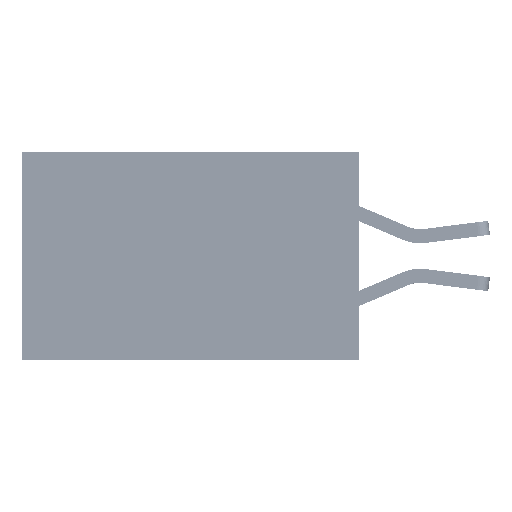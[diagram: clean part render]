
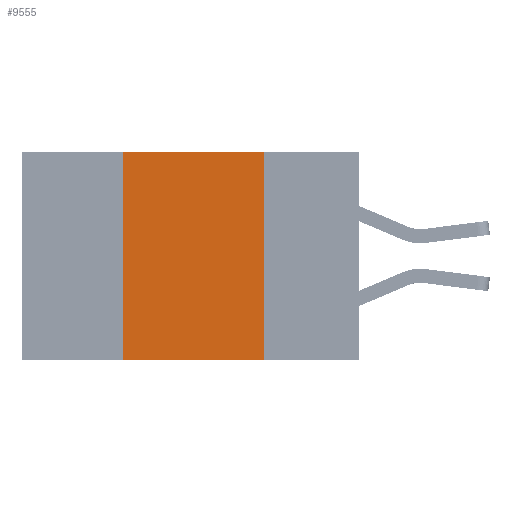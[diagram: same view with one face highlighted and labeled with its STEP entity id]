
A CAD part, left-side view. The second image highlights one B-rep face of the part: STEP entity #9555.
In plain terms, the highlighted planar face has unit normal (-1, 0, 0).
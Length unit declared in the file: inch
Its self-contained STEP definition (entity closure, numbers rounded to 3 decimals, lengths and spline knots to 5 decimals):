
#431 = VECTOR ( 'NONE', #17780, 39.37008 ) ;
#1274 = EDGE_CURVE ( 'NONE', #25482, #30341, #33294, .T. ) ;
#1359 = DIRECTION ( 'NONE',  ( 1., 0., 0. ) ) ;
#3663 = CARTESIAN_POINT ( 'NONE',  ( 0., 0.6, 0. ) ) ;
#5202 = EDGE_LOOP ( 'NONE', ( #25698, #6637, #6832, #24397 ) ) ;
#6637 = ORIENTED_EDGE ( 'NONE', *, *, #32102, .F. ) ;
#6832 = ORIENTED_EDGE ( 'NONE', *, *, #35600, .F. ) ;
#7669 = CARTESIAN_POINT ( 'NONE',  ( 0., 0.17, -0.37 ) ) ;
#7796 = VECTOR ( 'NONE', #33816, 39.37008 ) ;
#8931 = AXIS2_PLACEMENT_3D ( 'NONE', #3663, #1359, #23571 ) ;
#9555 = ADVANCED_FACE ( 'NONE', ( #10700 ), #32933, .F. ) ;
#10629 = VERTEX_POINT ( 'NONE', #11781 ) ;
#10692 = VECTOR ( 'NONE', #36409, 39.37008 ) ;
#10700 = FACE_OUTER_BOUND ( 'NONE', #5202, .T. ) ;
#11560 = LINE ( 'NONE', #14459, #431 ) ;
#11781 = CARTESIAN_POINT ( 'NONE',  ( 0., 0.42, -0.37 ) ) ;
#14459 = CARTESIAN_POINT ( 'NONE',  ( 0., 0.6, 0. ) ) ;
#14593 = CARTESIAN_POINT ( 'NONE',  ( 0., 0.17, 0. ) ) ;
#17780 = DIRECTION ( 'NONE',  ( 0., -1., 0. ) ) ;
#18869 = VERTEX_POINT ( 'NONE', #40530 ) ;
#23571 = DIRECTION ( 'NONE',  ( 0., 0., -1. ) ) ;
#24397 = ORIENTED_EDGE ( 'NONE', *, *, #39860, .T. ) ;
#25482 = VERTEX_POINT ( 'NONE', #27565 ) ;
#25698 = ORIENTED_EDGE ( 'NONE', *, *, #1274, .F. ) ;
#25746 = CARTESIAN_POINT ( 'NONE',  ( 0., 0.6, -0.37 ) ) ;
#27565 = CARTESIAN_POINT ( 'NONE',  ( 0., 0.17, 0. ) ) ;
#30341 = VERTEX_POINT ( 'NONE', #7669 ) ;
#31528 = CARTESIAN_POINT ( 'NONE',  ( 0., 0.42, 0. ) ) ;
#31774 = LINE ( 'NONE', #25746, #37896 ) ;
#31984 = DIRECTION ( 'NONE',  ( 0., -1., 0. ) ) ;
#32102 = EDGE_CURVE ( 'NONE', #18869, #25482, #11560, .T. ) ;
#32933 = PLANE ( 'NONE',  #8931 ) ;
#33294 = LINE ( 'NONE', #14593, #10692 ) ;
#33816 = DIRECTION ( 'NONE',  ( 0., 0., 1. ) ) ;
#35600 = EDGE_CURVE ( 'NONE', #10629, #18869, #37545, .T. ) ;
#36409 = DIRECTION ( 'NONE',  ( 0., 0., -1. ) ) ;
#37545 = LINE ( 'NONE', #31528, #7796 ) ;
#37896 = VECTOR ( 'NONE', #31984, 39.37008 ) ;
#39860 = EDGE_CURVE ( 'NONE', #10629, #30341, #31774, .T. ) ;
#40530 = CARTESIAN_POINT ( 'NONE',  ( 0., 0.42, 0. ) ) ;
